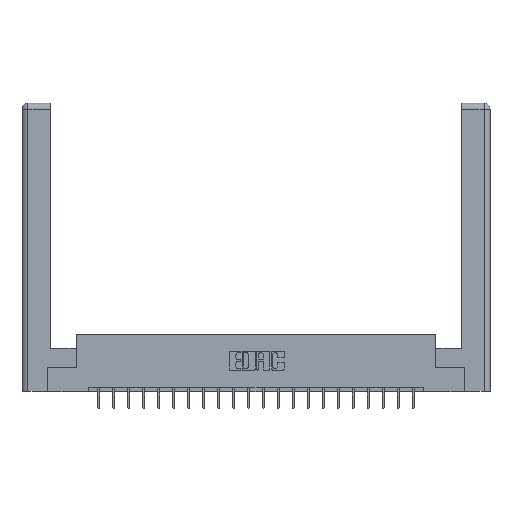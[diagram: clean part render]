
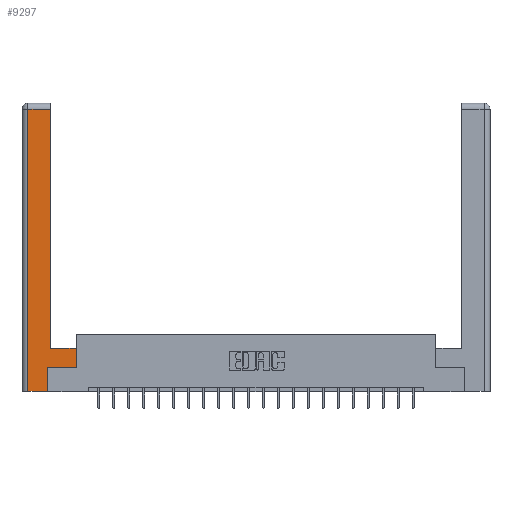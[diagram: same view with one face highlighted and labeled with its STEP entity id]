
A CAD part, top view. The second image highlights one B-rep face of the part: STEP entity #9297.
In plain terms, the highlighted planar face has unit normal (0, 0, 1).
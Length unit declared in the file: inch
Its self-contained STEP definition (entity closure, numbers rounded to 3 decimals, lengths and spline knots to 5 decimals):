
#249 = CARTESIAN_POINT ( 'NONE',  ( 0.565, 0.245, 0. ) ) ;
#398 = LINE ( 'NONE', #7568, #1480 ) ;
#846 = DIRECTION ( 'NONE',  ( 1., 0., 0. ) ) ;
#921 = PLANE ( 'NONE',  #2524 ) ;
#1265 = CARTESIAN_POINT ( 'NONE',  ( 0.565, 0.45, 0. ) ) ;
#1480 = VECTOR ( 'NONE', #846, 39.37008 ) ;
#2011 = CARTESIAN_POINT ( 'NONE',  ( 0.565, 0.245, 0. ) ) ;
#2364 = EDGE_LOOP ( 'NONE', ( #6478, #12662, #4689, #20694, #5218, #17560, #16727, #2387 ) ) ;
#2387 = ORIENTED_EDGE ( 'NONE', *, *, #14467, .T. ) ;
#2491 = CARTESIAN_POINT ( 'NONE',  ( 0.295, 0.45, 0. ) ) ;
#2524 = AXIS2_PLACEMENT_3D ( 'NONE', #12992, #11199, #2635 ) ;
#2605 = CARTESIAN_POINT ( 'NONE',  ( 0.265, 0., 0. ) ) ;
#2635 = DIRECTION ( 'NONE',  ( -1., 0., 0. ) ) ;
#2707 = DIRECTION ( 'NONE',  ( 0., -1., 0. ) ) ;
#2800 = DIRECTION ( 'NONE',  ( 0., 1., 0. ) ) ;
#3640 = CARTESIAN_POINT ( 'NONE',  ( 0.0615, 0., 0. ) ) ;
#3944 = EDGE_CURVE ( 'NONE', #20121, #12178, #20316, .T. ) ;
#4097 = VECTOR ( 'NONE', #22181, 39.37008 ) ;
#4214 = VECTOR ( 'NONE', #21095, 39.37008 ) ;
#4410 = CARTESIAN_POINT ( 'NONE',  ( 0.565, 0.45, 0. ) ) ;
#4689 = ORIENTED_EDGE ( 'NONE', *, *, #20544, .T. ) ;
#4756 = CARTESIAN_POINT ( 'NONE',  ( 0.295, 2.94, 0. ) ) ;
#4980 = CARTESIAN_POINT ( 'NONE',  ( 0.0615, 2.94, 0. ) ) ;
#5218 = ORIENTED_EDGE ( 'NONE', *, *, #3944, .T. ) ;
#5381 = LINE ( 'NONE', #2491, #6232 ) ;
#6232 = VECTOR ( 'NONE', #16326, 39.37008 ) ;
#6478 = ORIENTED_EDGE ( 'NONE', *, *, #18131, .T. ) ;
#6701 = CARTESIAN_POINT ( 'NONE',  ( 0.0615, 2.94, 0. ) ) ;
#7291 = VERTEX_POINT ( 'NONE', #4980 ) ;
#7349 = VERTEX_POINT ( 'NONE', #4756 ) ;
#7568 = CARTESIAN_POINT ( 'NONE',  ( 0.265, 0., 0. ) ) ;
#9055 = VERTEX_POINT ( 'NONE', #249 ) ;
#9257 = VECTOR ( 'NONE', #9643, 39.37008 ) ;
#9297 = ADVANCED_FACE ( 'NONE', ( #19147 ), #921, .F. ) ;
#9447 = CARTESIAN_POINT ( 'NONE',  ( 0.0615, 0., 0. ) ) ;
#9643 = DIRECTION ( 'NONE',  ( 0., 1., 0. ) ) ;
#10218 = VECTOR ( 'NONE', #2800, 39.37008 ) ;
#11199 = DIRECTION ( 'NONE',  ( 0., 0., -1. ) ) ;
#12178 = VERTEX_POINT ( 'NONE', #17942 ) ;
#12190 = VECTOR ( 'NONE', #16553, 39.37008 ) ;
#12662 = ORIENTED_EDGE ( 'NONE', *, *, #13966, .T. ) ;
#12992 = CARTESIAN_POINT ( 'NONE',  ( 0., 0., 0. ) ) ;
#13966 = EDGE_CURVE ( 'NONE', #7349, #7291, #16771, .T. ) ;
#14265 = EDGE_CURVE ( 'NONE', #9055, #14305, #21335, .T. ) ;
#14305 = VERTEX_POINT ( 'NONE', #4410 ) ;
#14467 = EDGE_CURVE ( 'NONE', #14305, #16028, #5381, .T. ) ;
#14639 = VECTOR ( 'NONE', #2707, 39.37008 ) ;
#15185 = LINE ( 'NONE', #9447, #14639 ) ;
#16028 = VERTEX_POINT ( 'NONE', #20476 ) ;
#16326 = DIRECTION ( 'NONE',  ( -1., 0., 0. ) ) ;
#16486 = CARTESIAN_POINT ( 'NONE',  ( 0.265, 0.245, 0. ) ) ;
#16553 = DIRECTION ( 'NONE',  ( 0., 1., 0. ) ) ;
#16727 = ORIENTED_EDGE ( 'NONE', *, *, #14265, .T. ) ;
#16771 = LINE ( 'NONE', #6701, #4097 ) ;
#17560 = ORIENTED_EDGE ( 'NONE', *, *, #18579, .T. ) ;
#17753 = LINE ( 'NONE', #18271, #10218 ) ;
#17942 = CARTESIAN_POINT ( 'NONE',  ( 0.265, 0.245, 0. ) ) ;
#18131 = EDGE_CURVE ( 'NONE', #16028, #7349, #17753, .T. ) ;
#18271 = CARTESIAN_POINT ( 'NONE',  ( 0.295, 3., 0. ) ) ;
#18579 = EDGE_CURVE ( 'NONE', #12178, #9055, #20959, .T. ) ;
#19147 = FACE_OUTER_BOUND ( 'NONE', #2364, .T. ) ;
#19776 = EDGE_CURVE ( 'NONE', #20327, #20121, #398, .T. ) ;
#20121 = VERTEX_POINT ( 'NONE', #2605 ) ;
#20316 = LINE ( 'NONE', #16486, #9257 ) ;
#20327 = VERTEX_POINT ( 'NONE', #3640 ) ;
#20476 = CARTESIAN_POINT ( 'NONE',  ( 0.295, 0.45, 0. ) ) ;
#20544 = EDGE_CURVE ( 'NONE', #7291, #20327, #15185, .T. ) ;
#20694 = ORIENTED_EDGE ( 'NONE', *, *, #19776, .T. ) ;
#20959 = LINE ( 'NONE', #2011, #4214 ) ;
#21095 = DIRECTION ( 'NONE',  ( 1., 0., 0. ) ) ;
#21335 = LINE ( 'NONE', #1265, #12190 ) ;
#22181 = DIRECTION ( 'NONE',  ( -1., 0., 0. ) ) ;
